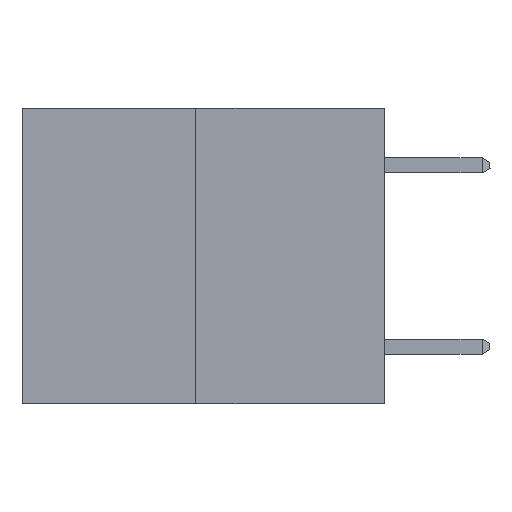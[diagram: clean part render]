
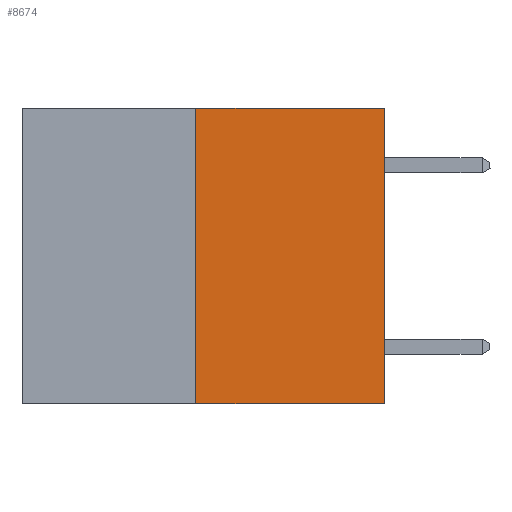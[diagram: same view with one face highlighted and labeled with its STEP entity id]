
A CAD part, left-side view. The second image highlights one B-rep face of the part: STEP entity #8674.
In plain terms, the highlighted planar face has unit normal (-1, 0, 0).
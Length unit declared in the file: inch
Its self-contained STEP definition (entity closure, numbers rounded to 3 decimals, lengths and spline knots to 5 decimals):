
#556 = LINE ( 'NONE', #16187, #10493 ) ;
#1117 = EDGE_CURVE ( 'NONE', #1590, #2754, #23751, .T. ) ;
#1136 = FACE_OUTER_BOUND ( 'NONE', #25602, .T. ) ;
#1590 = VERTEX_POINT ( 'NONE', #5902 ) ;
#1643 = DIRECTION ( 'NONE',  ( 0., 0., -1. ) ) ;
#2754 = VERTEX_POINT ( 'NONE', #24574 ) ;
#3729 = CARTESIAN_POINT ( 'NONE',  ( 0., 0.6, 0. ) ) ;
#4034 = DIRECTION ( 'NONE',  ( 1., 0., 0. ) ) ;
#4052 = VECTOR ( 'NONE', #8708, 39.37008 ) ;
#5902 = CARTESIAN_POINT ( 'NONE',  ( 0., 0., -0.49 ) ) ;
#7147 = CARTESIAN_POINT ( 'NONE',  ( 0., 0.312, 0. ) ) ;
#7606 = LINE ( 'NONE', #22243, #4052 ) ;
#8674 = ADVANCED_FACE ( 'NONE', ( #1136 ), #17384, .F. ) ;
#8708 = DIRECTION ( 'NONE',  ( 0., 0., 1. ) ) ;
#9755 = DIRECTION ( 'NONE',  ( 0., 0., 1. ) ) ;
#10493 = VECTOR ( 'NONE', #14013, 39.37008 ) ;
#11089 = ORIENTED_EDGE ( 'NONE', *, *, #27309, .F. ) ;
#12195 = VERTEX_POINT ( 'NONE', #7147 ) ;
#13102 = LINE ( 'NONE', #22952, #19512 ) ;
#14013 = DIRECTION ( 'NONE',  ( 0., -1., 0. ) ) ;
#16187 = CARTESIAN_POINT ( 'NONE',  ( 0., 0.6, 0. ) ) ;
#16235 = EDGE_CURVE ( 'NONE', #16282, #1590, #13102, .T. ) ;
#16282 = VERTEX_POINT ( 'NONE', #18612 ) ;
#16340 = DIRECTION ( 'NONE',  ( 0., -1., 0. ) ) ;
#16472 = CARTESIAN_POINT ( 'NONE',  ( 0., 0., 0. ) ) ;
#16563 = ORIENTED_EDGE ( 'NONE', *, *, #1117, .T. ) ;
#17384 = PLANE ( 'NONE',  #20922 ) ;
#18612 = CARTESIAN_POINT ( 'NONE',  ( 0., 0.312, -0.49 ) ) ;
#19512 = VECTOR ( 'NONE', #16340, 39.37008 ) ;
#20922 = AXIS2_PLACEMENT_3D ( 'NONE', #3729, #4034, #1643 ) ;
#21587 = VECTOR ( 'NONE', #9755, 39.37008 ) ;
#22243 = CARTESIAN_POINT ( 'NONE',  ( 0., 0.312, -0.49 ) ) ;
#22425 = ORIENTED_EDGE ( 'NONE', *, *, #22649, .F. ) ;
#22649 = EDGE_CURVE ( 'NONE', #16282, #12195, #7606, .T. ) ;
#22952 = CARTESIAN_POINT ( 'NONE',  ( 0., 0.6, -0.49 ) ) ;
#23751 = LINE ( 'NONE', #16472, #21587 ) ;
#24574 = CARTESIAN_POINT ( 'NONE',  ( 0., 0., 0. ) ) ;
#25602 = EDGE_LOOP ( 'NONE', ( #22425, #28633, #16563, #11089 ) ) ;
#27309 = EDGE_CURVE ( 'NONE', #12195, #2754, #556, .T. ) ;
#28633 = ORIENTED_EDGE ( 'NONE', *, *, #16235, .T. ) ;
